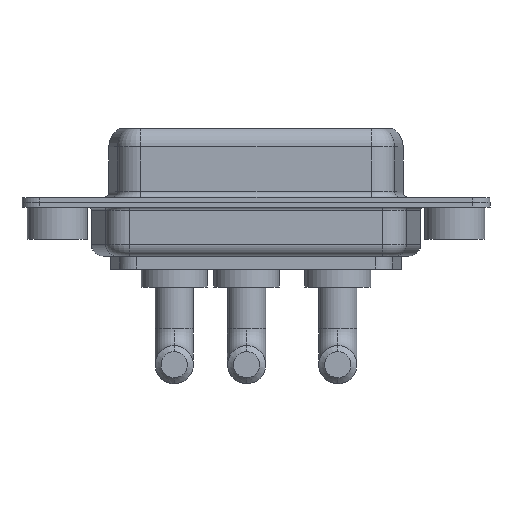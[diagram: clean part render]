
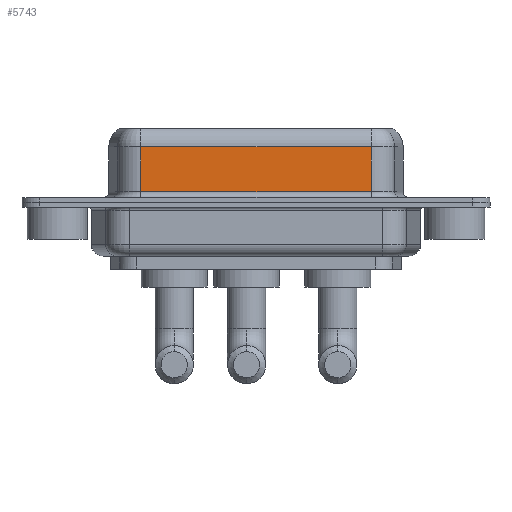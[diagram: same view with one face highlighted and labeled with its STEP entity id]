
A CAD part, front view. The second image highlights one B-rep face of the part: STEP entity #5743.
In plain terms, the highlighted planar face has unit normal (0, -1, 0).
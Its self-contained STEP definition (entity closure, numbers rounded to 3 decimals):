
#35 = FACE_OUTER_BOUND ( 'NONE', #4717, .T. ) ;
#129 = DIRECTION ( 'NONE',  ( 0., 0., -1. ) ) ;
#323 = LINE ( 'NONE', #8886, #11407 ) ;
#2673 = ORIENTED_EDGE ( 'NONE', *, *, #8656, .T. ) ;
#3258 = VERTEX_POINT ( 'NONE', #10459 ) ;
#3319 = LINE ( 'NONE', #10847, #12916 ) ;
#3811 = AXIS2_PLACEMENT_3D ( 'NONE', #8530, #12781, #11861 ) ;
#4264 = PLANE ( 'NONE',  #3811 ) ;
#4349 = ORIENTED_EDGE ( 'NONE', *, *, #5362, .F. ) ;
#4528 = CARTESIAN_POINT ( 'NONE',  ( 26.287, -3.95, 0.9 ) ) ;
#4717 = EDGE_LOOP ( 'NONE', ( #4349, #6885, #2673, #10744 ) ) ;
#5158 = VERTEX_POINT ( 'NONE', #7036 ) ;
#5336 = LINE ( 'NONE', #12919, #11430 ) ;
#5362 = EDGE_CURVE ( 'NONE', #7550, #6765, #3319, .T. ) ;
#5486 = CARTESIAN_POINT ( 'NONE',  ( 26.287, -3.95, 0.9 ) ) ;
#5743 = ADVANCED_FACE ( 'NONE', ( #35 ), #4264, .F. ) ;
#6131 = VECTOR ( 'NONE', #8719, 1000. ) ;
#6765 = VERTEX_POINT ( 'NONE', #5486 ) ;
#6885 = ORIENTED_EDGE ( 'NONE', *, *, #9340, .T. ) ;
#6934 = DIRECTION ( 'NONE',  ( 0., 0., -1. ) ) ;
#7036 = CARTESIAN_POINT ( 'NONE',  ( 7.013, -3.95, 0.9 ) ) ;
#7469 = LINE ( 'NONE', #4528, #6131 ) ;
#7550 = VERTEX_POINT ( 'NONE', #10806 ) ;
#8530 = CARTESIAN_POINT ( 'NONE',  ( 26.287, -3.95, 6.4 ) ) ;
#8656 = EDGE_CURVE ( 'NONE', #3258, #5158, #323, .T. ) ;
#8719 = DIRECTION ( 'NONE',  ( 1., 0., 0. ) ) ;
#8886 = CARTESIAN_POINT ( 'NONE',  ( 7.013, -3.95, 6.4 ) ) ;
#9340 = EDGE_CURVE ( 'NONE', #7550, #3258, #5336, .T. ) ;
#10459 = CARTESIAN_POINT ( 'NONE',  ( 7.013, -3.95, 4.65 ) ) ;
#10744 = ORIENTED_EDGE ( 'NONE', *, *, #11911, .T. ) ;
#10806 = CARTESIAN_POINT ( 'NONE',  ( 26.287, -3.95, 4.65 ) ) ;
#10847 = CARTESIAN_POINT ( 'NONE',  ( 26.287, -3.95, 6.4 ) ) ;
#10901 = DIRECTION ( 'NONE',  ( -1., 0., 0. ) ) ;
#11407 = VECTOR ( 'NONE', #6934, 1000. ) ;
#11430 = VECTOR ( 'NONE', #10901, 1000. ) ;
#11861 = DIRECTION ( 'NONE',  ( 0., 0., 1. ) ) ;
#11911 = EDGE_CURVE ( 'NONE', #5158, #6765, #7469, .T. ) ;
#12781 = DIRECTION ( 'NONE',  ( 0., 1., 0. ) ) ;
#12916 = VECTOR ( 'NONE', #129, 1000. ) ;
#12919 = CARTESIAN_POINT ( 'NONE',  ( 26.287, -3.95, 4.65 ) ) ;
